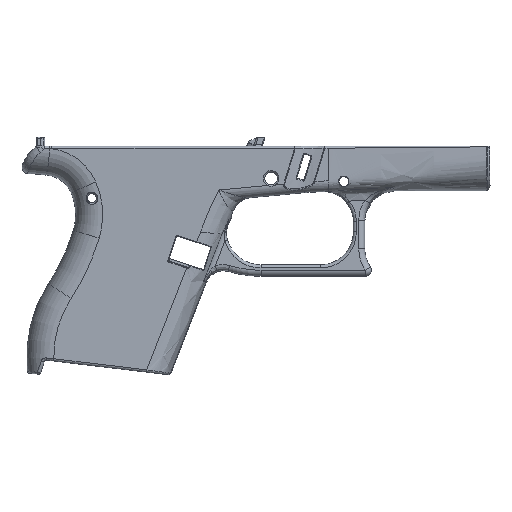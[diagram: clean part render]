
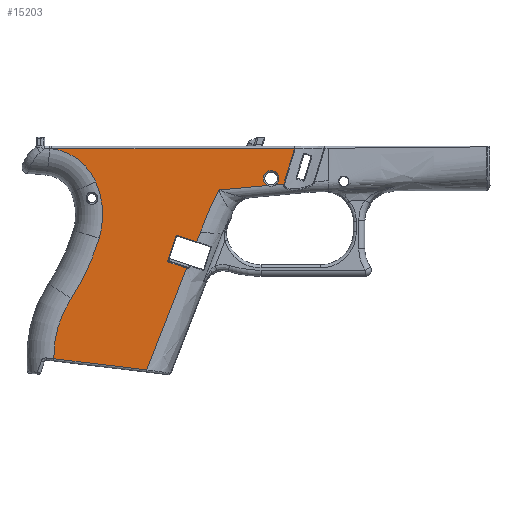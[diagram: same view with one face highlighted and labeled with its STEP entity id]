
A CAD part, front view. The second image highlights one B-rep face of the part: STEP entity #15203.
In plain terms, the highlighted planar face has unit normal (0, -1, 0).
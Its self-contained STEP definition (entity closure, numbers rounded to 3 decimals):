
#261=CIRCLE('',#15490,156.771);
#672=CIRCLE('',#16404,27.167);
#675=CIRCLE('',#16408,77.599);
#676=CIRCLE('',#16411,0.45);
#677=CIRCLE('',#16414,0.45);
#712=CIRCLE('',#16511,2.625);
#713=CIRCLE('',#16512,2.625);
#737=CIRCLE('',#16587,18.891);
#738=CIRCLE('',#16589,35.645);
#1265=LINE('',#23064,#2113);
#1267=LINE('',#23087,#2115);
#1814=LINE('',#39322,#2662);
#1817=LINE('',#39330,#2665);
#1819=LINE('',#39336,#2667);
#1886=LINE('',#39972,#2734);
#1933=LINE('',#42567,#2781);
#1934=LINE('',#42568,#2782);
#1935=LINE('',#42569,#2783);
#1936=LINE('',#42570,#2784);
#2113=VECTOR('',#17079,1000.);
#2115=VECTOR('',#17081,1000.);
#2662=VECTOR('',#19428,1000.);
#2665=VECTOR('',#19437,1000.);
#2667=VECTOR('',#19445,1000.);
#2734=VECTOR('',#19670,1000.);
#2781=VECTOR('',#19907,1000.);
#2782=VECTOR('',#19908,1000.);
#2783=VECTOR('',#19909,1000.);
#2784=VECTOR('',#19910,1000.);
#3242=PLANE('',#16588);
#3964=FACE_OUTER_BOUND('',#4903,.T.);
#4903=EDGE_LOOP('',(#13063,#13064,#13065,#13066,#13067,#13068,#13069,#13070,
#13071,#13072,#13073,#13074,#13075,#13076,#13077,#13078,#13079,#13080,#13081));
#5913=VERTEX_POINT('',#22254);
#5914=VERTEX_POINT('',#22343);
#5960=VERTEX_POINT('',#23062);
#5961=VERTEX_POINT('',#23063);
#5963=VERTEX_POINT('',#23086);
#6882=VERTEX_POINT('',#39310);
#6883=VERTEX_POINT('',#39312);
#6884=VERTEX_POINT('',#39316);
#6885=VERTEX_POINT('',#39320);
#6886=VERTEX_POINT('',#39324);
#6887=VERTEX_POINT('',#39328);
#6888=VERTEX_POINT('',#39332);
#6958=VERTEX_POINT('',#39969);
#6959=VERTEX_POINT('',#39971);
#6973=VERTEX_POINT('',#40179);
#6974=VERTEX_POINT('',#40181);
#6975=VERTEX_POINT('',#40183);
#7050=VERTEX_POINT('',#42561);
#7051=VERTEX_POINT('',#42565);
#7334=EDGE_CURVE('',#5914,#5913,#261,.T.);
#7385=EDGE_CURVE('',#5960,#5961,#1265,.F.);
#7389=EDGE_CURVE('',#5914,#5963,#1267,.F.);
#8865=EDGE_CURVE('',#6882,#6883,#672,.T.);
#8868=EDGE_CURVE('',#6884,#6882,#675,.T.);
#8870=EDGE_CURVE('',#6885,#5960,#1814,.T.);
#8872=EDGE_CURVE('',#6886,#6885,#676,.T.);
#8874=EDGE_CURVE('',#6887,#6886,#1817,.T.);
#8876=EDGE_CURVE('',#6888,#6887,#677,.T.);
#8877=EDGE_CURVE('',#5963,#6888,#1819,.T.);
#8994=EDGE_CURVE('',#6958,#6959,#1886,.T.);
#9022=EDGE_CURVE('',#6973,#6974,#712,.T.);
#9024=EDGE_CURVE('',#6975,#6973,#713,.T.);
#9148=EDGE_CURVE('',#6883,#7050,#737,.T.);
#9149=EDGE_CURVE('',#7051,#6884,#738,.T.);
#9150=EDGE_CURVE('',#7051,#5961,#1933,.F.);
#9151=EDGE_CURVE('',#6974,#5913,#1934,.T.);
#9152=EDGE_CURVE('',#6959,#6975,#1935,.T.);
#9153=EDGE_CURVE('',#7050,#6958,#1936,.T.);
#13063=ORIENTED_EDGE('',*,*,#9149,.F.);
#13064=ORIENTED_EDGE('',*,*,#9150,.T.);
#13065=ORIENTED_EDGE('',*,*,#7385,.F.);
#13066=ORIENTED_EDGE('',*,*,#8870,.F.);
#13067=ORIENTED_EDGE('',*,*,#8872,.F.);
#13068=ORIENTED_EDGE('',*,*,#8874,.F.);
#13069=ORIENTED_EDGE('',*,*,#8876,.F.);
#13070=ORIENTED_EDGE('',*,*,#8877,.F.);
#13071=ORIENTED_EDGE('',*,*,#7389,.F.);
#13072=ORIENTED_EDGE('',*,*,#7334,.T.);
#13073=ORIENTED_EDGE('',*,*,#9151,.F.);
#13074=ORIENTED_EDGE('',*,*,#9022,.F.);
#13075=ORIENTED_EDGE('',*,*,#9024,.F.);
#13076=ORIENTED_EDGE('',*,*,#9152,.F.);
#13077=ORIENTED_EDGE('',*,*,#8994,.F.);
#13078=ORIENTED_EDGE('',*,*,#9153,.F.);
#13079=ORIENTED_EDGE('',*,*,#9148,.F.);
#13080=ORIENTED_EDGE('',*,*,#8865,.F.);
#13081=ORIENTED_EDGE('',*,*,#8868,.F.);
#15203=ADVANCED_FACE('',(#3964),#3242,.T.);
#15490=AXIS2_PLACEMENT_3D('',#22344,#17030,#17031);
#16404=AXIS2_PLACEMENT_3D('',#39313,#19415,#19416);
#16408=AXIS2_PLACEMENT_3D('',#39318,#19423,#19424);
#16411=AXIS2_PLACEMENT_3D('',#39326,#19432,#19433);
#16414=AXIS2_PLACEMENT_3D('',#39334,#19441,#19442);
#16511=AXIS2_PLACEMENT_3D('',#40182,#19717,#19718);
#16512=AXIS2_PLACEMENT_3D('',#40194,#19719,#19720);
#16587=AXIS2_PLACEMENT_3D('',#42563,#19901,#19902);
#16588=AXIS2_PLACEMENT_3D('',#42564,#19903,#19904);
#16589=AXIS2_PLACEMENT_3D('',#42566,#19905,#19906);
#17030=DIRECTION('center_axis',(0.,1.,0.));
#17031=DIRECTION('ref_axis',(-0.937,0.,0.35));
#17079=DIRECTION('',(0.363,0.,0.932));
#17081=DIRECTION('',(0.363,0.,0.932));
#19415=DIRECTION('center_axis',(0.,-1.,0.));
#19416=DIRECTION('ref_axis',(0.998,0.,0.06));
#19423=DIRECTION('center_axis',(0.,-1.,0.));
#19424=DIRECTION('ref_axis',(0.907,0.,-0.421));
#19428=DIRECTION('',(0.951,0.,-0.309));
#19432=DIRECTION('center_axis',(0.,-1.,0.));
#19433=DIRECTION('ref_axis',(-0.891,0.,-0.454));
#19437=DIRECTION('',(-0.309,0.,-0.951));
#19441=DIRECTION('center_axis',(0.,-1.,0.));
#19442=DIRECTION('ref_axis',(-0.454,0.,0.891));
#19445=DIRECTION('',(-0.951,0.,0.309));
#19670=DIRECTION('',(-0.292,0.,-0.956));
#19717=DIRECTION('center_axis',(0.,-1.,0.));
#19718=DIRECTION('ref_axis',(-1.,0.,0.));
#19719=DIRECTION('center_axis',(0.,-1.,0.));
#19720=DIRECTION('ref_axis',(-1.,0.,0.));
#19901=DIRECTION('center_axis',(0.,-1.,0.));
#19902=DIRECTION('ref_axis',(0.592,0.,0.806));
#19903=DIRECTION('center_axis',(0.,-1.,0.));
#19904=DIRECTION('ref_axis',(1.,0.,0.));
#19905=DIRECTION('center_axis',(0.,1.,0.));
#19906=DIRECTION('ref_axis',(-0.961,0.,0.276));
#19907=DIRECTION('',(-0.993,0.,0.119));
#19908=DIRECTION('',(-0.996,0.,-0.092));
#19909=DIRECTION('',(-0.996,0.,-0.092));
#19910=DIRECTION('',(1.,0.,0.));
#22254=CARTESIAN_POINT('',(-14.141,-11.5,11.929));
#22343=CARTESIAN_POINT('',(-20.166,-11.5,-2.06));
#22344=CARTESIAN_POINT('Origin',(126.663,-11.5,-57.001));
#23062=CARTESIAN_POINT('',(-24.83,-11.5,-14.036));
#23063=CARTESIAN_POINT('',(-38.041,-11.5,-47.95));
#23064=CARTESIAN_POINT('',(-29.536,-11.5,-26.116));
#23086=CARTESIAN_POINT('',(-21.413,-11.5,-5.263));
#23087=CARTESIAN_POINT('',(-20.166,-11.5,-2.06));
#39310=CARTESIAN_POINT('',(-53.881,-11.5,-4.09));
#39312=CARTESIAN_POINT('',(-55.002,-11.5,14.602));
#39313=CARTESIAN_POINT('Origin',(-79.899,-11.5,3.729));
#39316=CARTESIAN_POINT('',(-63.213,-11.5,-24.169));
#39318=CARTESIAN_POINT('Origin',(-128.196,-11.5,18.243));
#39320=CARTESIAN_POINT('',(-30.68,-11.5,-12.136));
#39322=CARTESIAN_POINT('',(-14.586,-11.5,-17.365));
#39324=CARTESIAN_POINT('',(-30.968,-11.5,-11.569));
#39326=CARTESIAN_POINT('Origin',(-30.54,-11.5,-11.708));
#39328=CARTESIAN_POINT('',(-28.342,-11.5,-3.485));
#39330=CARTESIAN_POINT('',(-28.119,-11.5,-2.799));
#39332=CARTESIAN_POINT('',(-27.775,-11.5,-3.196));
#39334=CARTESIAN_POINT('Origin',(-27.914,-11.5,-3.624));
#39336=CARTESIAN_POINT('',(-9.303,-11.5,-9.197));
#39969=CARTESIAN_POINT('',(11.185,-11.5,25.75));
#39971=CARTESIAN_POINT('',(7.57,-11.5,13.924));
#39972=CARTESIAN_POINT('',(5.553,-11.5,7.328));
#40179=CARTESIAN_POINT('',(5.968,-11.5,15.788));
#40181=CARTESIAN_POINT('',(2.19,-11.5,13.43));
#40182=CARTESIAN_POINT('Origin',(3.343,-11.5,15.788));
#40183=CARTESIAN_POINT('',(4.906,-11.5,13.679));
#40194=CARTESIAN_POINT('Origin',(3.343,-11.5,15.788));
#42561=CARTESIAN_POINT('',(-69.695,-11.5,25.75));
#42563=CARTESIAN_POINT('Origin',(-72.315,-11.5,7.041));
#42564=CARTESIAN_POINT('Origin',(-1.777,-11.5,-10.863));
#42565=CARTESIAN_POINT('',(-69.003,-11.5,-44.245));
#42566=CARTESIAN_POINT('Origin',(-33.363,-11.5,-43.651));
#42567=CARTESIAN_POINT('',(-6.665,-11.5,-51.705));
#42568=CARTESIAN_POINT('',(4.861,-11.5,13.675));
#42569=CARTESIAN_POINT('',(4.861,-11.5,13.675));
#42570=CARTESIAN_POINT('',(37.236,-11.5,25.75));
